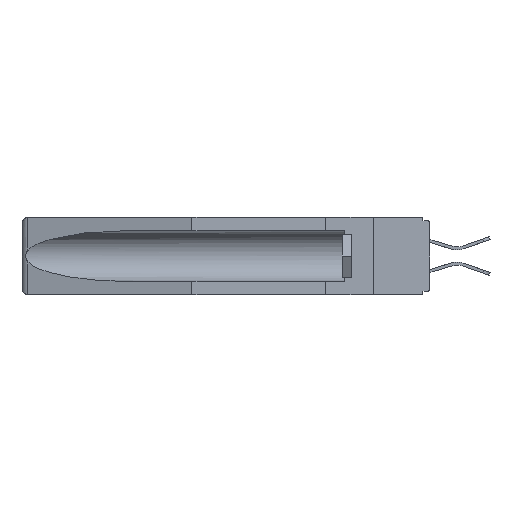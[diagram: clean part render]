
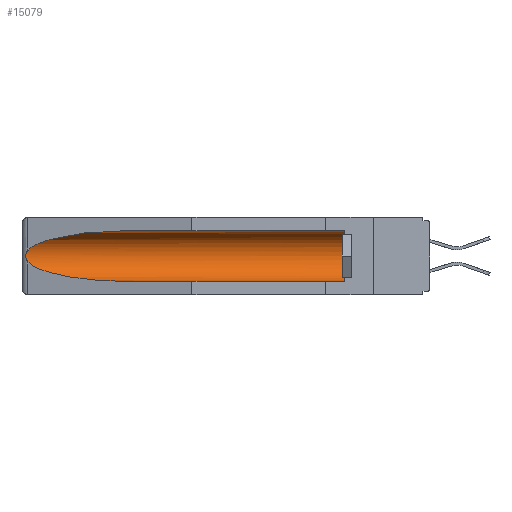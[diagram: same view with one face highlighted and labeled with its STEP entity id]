
A CAD part, left-side view. The second image highlights one B-rep face of the part: STEP entity #15079.
In plain terms, the highlighted cylindrical face has radius 2.857 mm (diameter 5.715 mm), a partial arc.
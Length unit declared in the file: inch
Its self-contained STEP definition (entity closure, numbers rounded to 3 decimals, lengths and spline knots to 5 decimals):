
#142 = EDGE_CURVE ( 'NONE', #13779, #18768, #8928, .T. ) ;
#328 = CARTESIAN_POINT ( 'NONE',  ( 0.21114, 1.30732, -0.284 ) ) ;
#381 = CARTESIAN_POINT ( 'NONE',  ( 0.2675, 1.53308, -0.17534 ) ) ;
#507 = CARTESIAN_POINT ( 'NONE',  ( 0.155, 0.126, -0.059 ) ) ;
#528 = CARTESIAN_POINT ( 'NONE',  ( 0.26537, 1.52718, -0.19328 ) ) ;
#890 = CARTESIAN_POINT ( 'NONE',  ( 0.155, 0.126, -0.1715 ) ) ;
#1681 = ORIENTED_EDGE ( 'NONE', *, *, #142, .T. ) ;
#2014 = LINE ( 'NONE', #7240, #18503 ) ;
#2183 = CARTESIAN_POINT ( 'NONE',  ( 0.2675, 1.53308, -0.16763 ) ) ;
#2320 = CYLINDRICAL_SURFACE ( 'NONE', #21059, 0.1125 ) ;
#2426 = EDGE_CURVE ( 'NONE', #10063, #22972, #2014, .T. ) ;
#3443 = CIRCLE ( 'NONE', #16705, 0.1125 ) ;
#4704 =( BOUNDED_CURVE ( )  B_SPLINE_CURVE ( 3, ( #14659, #7464, #328, #5543 ),
 .UNSPECIFIED., .F., .F. ) 
 B_SPLINE_CURVE_WITH_KNOTS ( ( 4, 4 ),
 ( 0.1948, 1.5708 ),
 .UNSPECIFIED. ) 
 CURVE ( )  GEOMETRIC_REPRESENTATION_ITEM ( )  RATIONAL_B_SPLINE_CURVE ( ( 1., 0.848, 0.848, 1. ) ) 
 REPRESENTATION_ITEM ( '' )  );
#5543 = CARTESIAN_POINT ( 'NONE',  ( 0.155, 1.07973, -0.284 ) ) ;
#5676 = CARTESIAN_POINT ( 'NONE',  ( 0.26597, 1.5296, -0.19026 ) ) ;
#5725 = FACE_OUTER_BOUND ( 'NONE', #18844, .T. ) ;
#5907 = CARTESIAN_POINT ( 'NONE',  ( 0.2673, 1.53269, -0.17917 ) ) ;
#7240 = CARTESIAN_POINT ( 'NONE',  ( 0.155, -0.30754, -0.284 ) ) ;
#7464 = CARTESIAN_POINT ( 'NONE',  ( 0.25451, 1.48313, -0.24835 ) ) ;
#8580 = CARTESIAN_POINT ( 'NONE',  ( 0.21114, 1.30732, -0.059 ) ) ;
#8724 = ORIENTED_EDGE ( 'NONE', *, *, #9888, .T. ) ;
#8928 =( BOUNDED_CURVE ( )  B_SPLINE_CURVE ( 3, ( #10006, #8580, #19123, #23247 ),
 .UNSPECIFIED., .F., .F. ) 
 B_SPLINE_CURVE_WITH_KNOTS ( ( 4, 4 ),
 ( 4.71239, 6.08839 ),
 .UNSPECIFIED. ) 
 CURVE ( )  GEOMETRIC_REPRESENTATION_ITEM ( )  RATIONAL_B_SPLINE_CURVE ( ( 1., 0.848, 0.848, 1. ) ) 
 REPRESENTATION_ITEM ( '' )  );
#9105 = DIRECTION ( 'NONE',  ( 0., 1., 0. ) ) ;
#9255 = CARTESIAN_POINT ( 'NONE',  ( 0.26597, 1.52961, -0.15275 ) ) ;
#9414 = CARTESIAN_POINT ( 'NONE',  ( 0.2673, 1.5327, -0.16383 ) ) ;
#9779 = EDGE_CURVE ( 'NONE', #22793, #22972, #4704, .T. ) ;
#9888 = EDGE_CURVE ( 'NONE', #10063, #22629, #3443, .T. ) ;
#9913 = CARTESIAN_POINT ( 'NONE',  ( 0.155, -0.30754, -0.1715 ) ) ;
#10006 = CARTESIAN_POINT ( 'NONE',  ( 0.155, 1.07973, -0.059 ) ) ;
#10063 = VERTEX_POINT ( 'NONE', #21710 ) ;
#11135 = ORIENTED_EDGE ( 'NONE', *, *, #9779, .T. ) ;
#12765 = EDGE_CURVE ( 'NONE', #18768, #22793, #21196, .T. ) ;
#13779 = VERTEX_POINT ( 'NONE', #15542 ) ;
#14659 = CARTESIAN_POINT ( 'NONE',  ( 0.26537, 1.52718, -0.19328 ) ) ;
#14942 = ORIENTED_EDGE ( 'NONE', *, *, #2426, .F. ) ;
#15079 = ADVANCED_FACE ( 'NONE', ( #5725 ), #2320, .F. ) ;
#15542 = CARTESIAN_POINT ( 'NONE',  ( 0.155, 1.07973, -0.059 ) ) ;
#15970 = CARTESIAN_POINT ( 'NONE',  ( 0.26537, 1.52718, -0.14972 ) ) ;
#16238 = DIRECTION ( 'NONE',  ( 0., 1., 0. ) ) ;
#16302 = CARTESIAN_POINT ( 'NONE',  ( 0.26537, 1.52718, -0.19328 ) ) ;
#16537 = CARTESIAN_POINT ( 'NONE',  ( 0.155, 1.07973, -0.284 ) ) ;
#16705 = AXIS2_PLACEMENT_3D ( 'NONE', #890, #20845, #20775 ) ;
#16815 = CARTESIAN_POINT ( 'NONE',  ( 0.26537, 1.52718, -0.14972 ) ) ;
#17610 = EDGE_CURVE ( 'NONE', #22629, #13779, #19109, .T. ) ;
#18435 = CARTESIAN_POINT ( 'NONE',  ( 0.26654, 1.53092, -0.15636 ) ) ;
#18503 = VECTOR ( 'NONE', #16238, 39.37008 ) ;
#18768 = VERTEX_POINT ( 'NONE', #15970 ) ;
#18844 = EDGE_LOOP ( 'NONE', ( #1681, #22482, #11135, #14942, #8724, #21053 ) ) ;
#19019 = DIRECTION ( 'NONE',  ( 0., 0., 1. ) ) ;
#19109 = LINE ( 'NONE', #20288, #20815 ) ;
#19123 = CARTESIAN_POINT ( 'NONE',  ( 0.25451, 1.48313, -0.09465 ) ) ;
#20288 = CARTESIAN_POINT ( 'NONE',  ( 0.155, -0.30754, -0.059 ) ) ;
#20775 = DIRECTION ( 'NONE',  ( 0., 0., 1. ) ) ;
#20815 = VECTOR ( 'NONE', #9105, 39.37008 ) ;
#20845 = DIRECTION ( 'NONE',  ( 0., -1., 0. ) ) ;
#21053 = ORIENTED_EDGE ( 'NONE', *, *, #17610, .T. ) ;
#21059 = AXIS2_PLACEMENT_3D ( 'NONE', #9913, #22684, #19019 ) ;
#21196 = B_SPLINE_CURVE_WITH_KNOTS ( 'NONE', 3,
 ( #16815, #9255, #18435, #9414, #2183, #381, #5907, #22002, #5676, #528 ),
 .UNSPECIFIED., .F., .F.,
 ( 4, 2, 2, 2, 4 ),
 ( 0., 0.00029, 0.00058, 0.00087, 0.00117 ),
 .UNSPECIFIED. ) ;
#21710 = CARTESIAN_POINT ( 'NONE',  ( 0.155, 0.126, -0.284 ) ) ;
#22002 = CARTESIAN_POINT ( 'NONE',  ( 0.26655, 1.53094, -0.18657 ) ) ;
#22482 = ORIENTED_EDGE ( 'NONE', *, *, #12765, .T. ) ;
#22629 = VERTEX_POINT ( 'NONE', #507 ) ;
#22684 = DIRECTION ( 'NONE',  ( 0., 1., 0. ) ) ;
#22793 = VERTEX_POINT ( 'NONE', #16302 ) ;
#22972 = VERTEX_POINT ( 'NONE', #16537 ) ;
#23247 = CARTESIAN_POINT ( 'NONE',  ( 0.26537, 1.52718, -0.14972 ) ) ;
